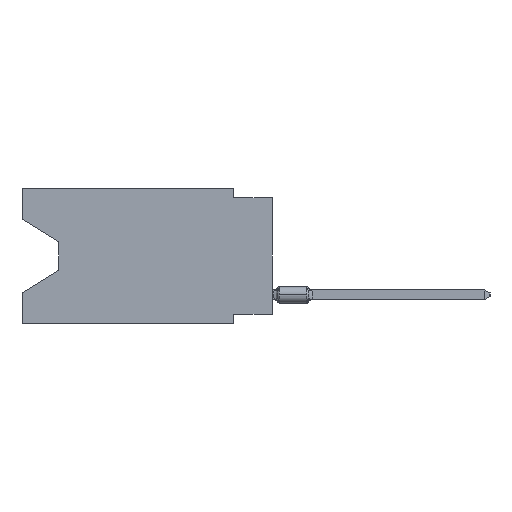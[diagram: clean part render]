
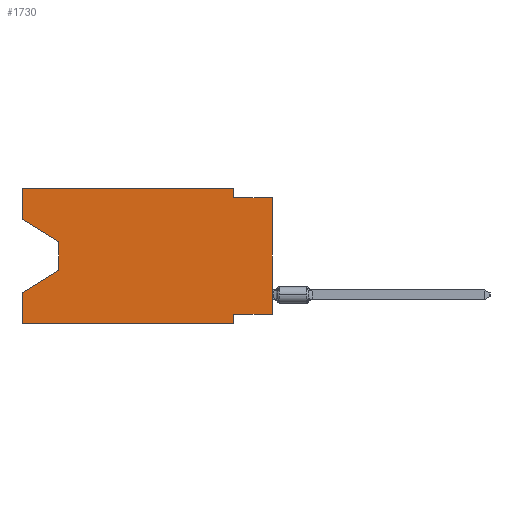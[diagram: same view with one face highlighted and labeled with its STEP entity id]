
A CAD part, left-side view. The second image highlights one B-rep face of the part: STEP entity #1730.
In plain terms, the highlighted planar face has unit normal (-1, 0, 0).
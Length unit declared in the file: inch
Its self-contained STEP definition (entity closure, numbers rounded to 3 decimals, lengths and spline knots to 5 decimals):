
#313 = VERTEX_POINT ( 'NONE', #26428 ) ;
#347 = VECTOR ( 'NONE', #12360, 39.37008 ) ;
#466 = ORIENTED_EDGE ( 'NONE', *, *, #7288, .T. ) ;
#1365 = LINE ( 'NONE', #13681, #9206 ) ;
#1665 = LINE ( 'NONE', #14620, #20029 ) ;
#1715 = ORIENTED_EDGE ( 'NONE', *, *, #10962, .T. ) ;
#1730 = ADVANCED_FACE ( 'NONE', ( #5330 ), #15213, .F. ) ;
#2037 = EDGE_CURVE ( 'NONE', #22505, #24113, #11469, .T. ) ;
#2191 = LINE ( 'NONE', #31852, #7097 ) ;
#2250 = LINE ( 'NONE', #5311, #28958 ) ;
#2408 = EDGE_CURVE ( 'NONE', #24881, #313, #2250, .T. ) ;
#2596 = DIRECTION ( 'NONE',  ( 0., 0., -1. ) ) ;
#2655 = ORIENTED_EDGE ( 'NONE', *, *, #2037, .F. ) ;
#2851 = EDGE_LOOP ( 'NONE', ( #7813, #11111, #466, #2655, #24195, #17058, #18317, #1715, #13139, #27133, #5533, #27492 ) ) ;
#3223 = CARTESIAN_POINT ( 'NONE',  ( 0., 0.645, 0. ) ) ;
#3645 = CARTESIAN_POINT ( 'NONE',  ( 0., 0.55, -0.212 ) ) ;
#4711 = CARTESIAN_POINT ( 'NONE',  ( 0., 0., 0. ) ) ;
#5311 = CARTESIAN_POINT ( 'NONE',  ( 0., 0.1, 0. ) ) ;
#5330 = FACE_OUTER_BOUND ( 'NONE', #2851, .T. ) ;
#5533 = ORIENTED_EDGE ( 'NONE', *, *, #20752, .F. ) ;
#6551 = DIRECTION ( 'NONE',  ( 0., -1., 0. ) ) ;
#7097 = VECTOR ( 'NONE', #14812, 39.37008 ) ;
#7288 = EDGE_CURVE ( 'NONE', #20767, #24113, #8786, .T. ) ;
#7813 = ORIENTED_EDGE ( 'NONE', *, *, #8515, .T. ) ;
#8515 = EDGE_CURVE ( 'NONE', #29991, #20142, #31419, .T. ) ;
#8786 = LINE ( 'NONE', #26767, #12633 ) ;
#9206 = VECTOR ( 'NONE', #18703, 39.37008 ) ;
#9650 = VERTEX_POINT ( 'NONE', #26089 ) ;
#9811 = VERTEX_POINT ( 'NONE', #28843 ) ;
#10086 = CARTESIAN_POINT ( 'NONE',  ( 0., 0.645, -0.26975 ) ) ;
#10599 = EDGE_CURVE ( 'NONE', #29991, #9650, #2191, .T. ) ;
#10621 = VECTOR ( 'NONE', #14710, 39.37008 ) ;
#10962 = EDGE_CURVE ( 'NONE', #29108, #9811, #12630, .T. ) ;
#11111 = ORIENTED_EDGE ( 'NONE', *, *, #24360, .T. ) ;
#11469 = LINE ( 'NONE', #21355, #31551 ) ;
#12165 = CARTESIAN_POINT ( 'NONE',  ( 0., 0.55, -0.138 ) ) ;
#12360 = DIRECTION ( 'NONE',  ( 0., 0., -1. ) ) ;
#12567 = CARTESIAN_POINT ( 'NONE',  ( 0., 0.1, 0. ) ) ;
#12630 = LINE ( 'NONE', #4711, #28715 ) ;
#12633 = VECTOR ( 'NONE', #13639, 39.37008 ) ;
#12663 = LINE ( 'NONE', #20433, #24340 ) ;
#12825 = EDGE_CURVE ( 'NONE', #29108, #15656, #12663, .T. ) ;
#13139 = ORIENTED_EDGE ( 'NONE', *, *, #14250, .F. ) ;
#13639 = DIRECTION ( 'NONE',  ( 0., 0.855, -0.519 ) ) ;
#13681 = CARTESIAN_POINT ( 'NONE',  ( 0., 0.645, 0. ) ) ;
#13869 = CARTESIAN_POINT ( 'NONE',  ( 0., 0.1, -0.325 ) ) ;
#13886 = VECTOR ( 'NONE', #6551, 39.37008 ) ;
#14166 = CARTESIAN_POINT ( 'NONE',  ( 0., 0.645, -0.35 ) ) ;
#14250 = EDGE_CURVE ( 'NONE', #313, #9811, #31891, .T. ) ;
#14383 = CARTESIAN_POINT ( 'NONE',  ( 0., 0., -0.025 ) ) ;
#14620 = CARTESIAN_POINT ( 'NONE',  ( 0., 0.55, -0.138 ) ) ;
#14710 = DIRECTION ( 'NONE',  ( 0., -0.855, -0.519 ) ) ;
#14812 = DIRECTION ( 'NONE',  ( 0., 0., 1. ) ) ;
#14879 = DIRECTION ( 'NONE',  ( 0., 0., -1. ) ) ;
#14947 = DIRECTION ( 'NONE',  ( 0., 1., 0. ) ) ;
#15213 = PLANE ( 'NONE',  #21662 ) ;
#15656 = VERTEX_POINT ( 'NONE', #13869 ) ;
#16089 = VERTEX_POINT ( 'NONE', #21042 ) ;
#16417 = CARTESIAN_POINT ( 'NONE',  ( 0., 0., -0.325 ) ) ;
#16654 = DIRECTION ( 'NONE',  ( 0., -1., 0. ) ) ;
#16686 = CARTESIAN_POINT ( 'NONE',  ( 0., 0.645, -0.35 ) ) ;
#16748 = LINE ( 'NONE', #29239, #347 ) ;
#16755 = LINE ( 'NONE', #14166, #13886 ) ;
#17058 = ORIENTED_EDGE ( 'NONE', *, *, #20921, .F. ) ;
#18317 = ORIENTED_EDGE ( 'NONE', *, *, #12825, .F. ) ;
#18703 = DIRECTION ( 'NONE',  ( 0., -1., 0. ) ) ;
#19038 = VECTOR ( 'NONE', #16654, 39.37008 ) ;
#19093 = CARTESIAN_POINT ( 'NONE',  ( 0., 0.645, -0.08025 ) ) ;
#20029 = VECTOR ( 'NONE', #24508, 39.37008 ) ;
#20142 = VERTEX_POINT ( 'NONE', #12165 ) ;
#20433 = CARTESIAN_POINT ( 'NONE',  ( 0., 0., -0.325 ) ) ;
#20752 = EDGE_CURVE ( 'NONE', #9650, #24881, #1365, .T. ) ;
#20767 = VERTEX_POINT ( 'NONE', #3645 ) ;
#20921 = EDGE_CURVE ( 'NONE', #15656, #16089, #16748, .T. ) ;
#21042 = CARTESIAN_POINT ( 'NONE',  ( 0., 0.1, -0.35 ) ) ;
#21355 = CARTESIAN_POINT ( 'NONE',  ( 0., 0.645, 0. ) ) ;
#21662 = AXIS2_PLACEMENT_3D ( 'NONE', #3223, #24797, #2596 ) ;
#22505 = VERTEX_POINT ( 'NONE', #16686 ) ;
#24113 = VERTEX_POINT ( 'NONE', #10086 ) ;
#24195 = ORIENTED_EDGE ( 'NONE', *, *, #27401, .T. ) ;
#24340 = VECTOR ( 'NONE', #14947, 39.37008 ) ;
#24360 = EDGE_CURVE ( 'NONE', #20142, #20767, #1665, .T. ) ;
#24508 = DIRECTION ( 'NONE',  ( 0., 0., -1. ) ) ;
#24797 = DIRECTION ( 'NONE',  ( 1., 0., 0. ) ) ;
#24881 = VERTEX_POINT ( 'NONE', #12567 ) ;
#26089 = CARTESIAN_POINT ( 'NONE',  ( 0., 0.645, 0. ) ) ;
#26248 = CARTESIAN_POINT ( 'NONE',  ( 0., 0.645, -0.08025 ) ) ;
#26428 = CARTESIAN_POINT ( 'NONE',  ( 0., 0.1, -0.025 ) ) ;
#26767 = CARTESIAN_POINT ( 'NONE',  ( 0., 0.55, -0.212 ) ) ;
#27133 = ORIENTED_EDGE ( 'NONE', *, *, #2408, .F. ) ;
#27343 = DIRECTION ( 'NONE',  ( 0., 0., 1. ) ) ;
#27401 = EDGE_CURVE ( 'NONE', #22505, #16089, #16755, .T. ) ;
#27492 = ORIENTED_EDGE ( 'NONE', *, *, #10599, .F. ) ;
#28715 = VECTOR ( 'NONE', #29665, 39.37008 ) ;
#28843 = CARTESIAN_POINT ( 'NONE',  ( 0., 0., -0.025 ) ) ;
#28958 = VECTOR ( 'NONE', #14879, 39.37008 ) ;
#29108 = VERTEX_POINT ( 'NONE', #16417 ) ;
#29239 = CARTESIAN_POINT ( 'NONE',  ( 0., 0.1, -0.35 ) ) ;
#29665 = DIRECTION ( 'NONE',  ( 0., 0., 1. ) ) ;
#29991 = VERTEX_POINT ( 'NONE', #26248 ) ;
#31419 = LINE ( 'NONE', #19093, #10621 ) ;
#31551 = VECTOR ( 'NONE', #27343, 39.37008 ) ;
#31852 = CARTESIAN_POINT ( 'NONE',  ( 0., 0.645, 0. ) ) ;
#31891 = LINE ( 'NONE', #14383, #19038 ) ;
